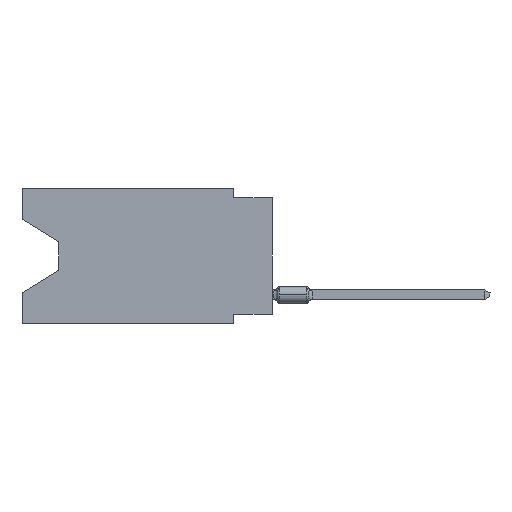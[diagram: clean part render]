
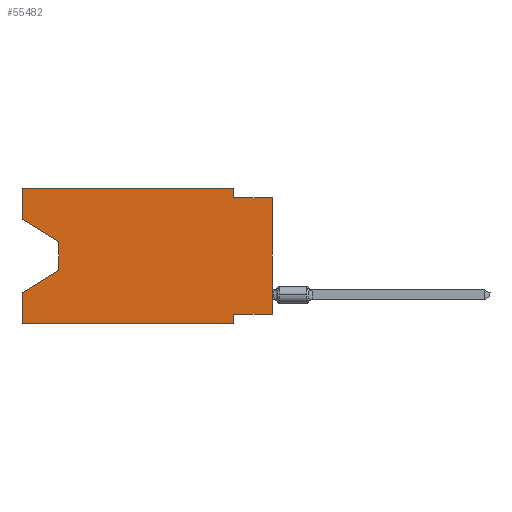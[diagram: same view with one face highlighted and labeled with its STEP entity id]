
A CAD part, left-side view. The second image highlights one B-rep face of the part: STEP entity #55482.
In plain terms, the highlighted planar face has unit normal (-1, 0, 0).
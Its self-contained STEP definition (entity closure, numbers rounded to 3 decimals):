
#681 = DIRECTION ( 'NONE',  ( 0., 0., -1. ) ) ;
#795 = CARTESIAN_POINT ( 'NONE',  ( 0., 16.383, 0. ) ) ;
#1353 = CARTESIAN_POINT ( 'NONE',  ( 0., 0., -0.635 ) ) ;
#1984 = EDGE_CURVE ( 'NONE', #32565, #71224, #25926, .T. ) ;
#2244 = CARTESIAN_POINT ( 'NONE',  ( 0., 16.383, 0. ) ) ;
#2328 = EDGE_LOOP ( 'NONE', ( #21225, #4674, #35212, #48874, #58972, #5348, #60784, #5587, #52796, #24719, #15482, #45468 ) ) ;
#2880 = CARTESIAN_POINT ( 'NONE',  ( 0., 2.54, -0.635 ) ) ;
#2923 = VERTEX_POINT ( 'NONE', #56044 ) ;
#3989 = CARTESIAN_POINT ( 'NONE',  ( 0., 16.383, -6.852 ) ) ;
#4352 = CARTESIAN_POINT ( 'NONE',  ( 0., 0., -8.255 ) ) ;
#4555 = CARTESIAN_POINT ( 'NONE',  ( 0., 16.383, -2.038 ) ) ;
#4674 = ORIENTED_EDGE ( 'NONE', *, *, #30506, .T. ) ;
#4693 = LINE ( 'NONE', #9456, #6741 ) ;
#5130 = VERTEX_POINT ( 'NONE', #795 ) ;
#5348 = ORIENTED_EDGE ( 'NONE', *, *, #31279, .F. ) ;
#5587 = ORIENTED_EDGE ( 'NONE', *, *, #11384, .T. ) ;
#5740 = VERTEX_POINT ( 'NONE', #2880 ) ;
#6534 = VECTOR ( 'NONE', #47181, 1000. ) ;
#6741 = VECTOR ( 'NONE', #36923, 1000. ) ;
#7385 = DIRECTION ( 'NONE',  ( 0., -1., 0. ) ) ;
#7559 = LINE ( 'NONE', #56991, #9021 ) ;
#7569 = LINE ( 'NONE', #13766, #56932 ) ;
#8771 = EDGE_CURVE ( 'NONE', #2923, #70282, #7569, .T. ) ;
#9021 = VECTOR ( 'NONE', #58058, 1000. ) ;
#9230 = EDGE_CURVE ( 'NONE', #18160, #30103, #10346, .T. ) ;
#9456 = CARTESIAN_POINT ( 'NONE',  ( 0., 0., 0. ) ) ;
#9576 = EDGE_CURVE ( 'NONE', #5130, #12371, #41776, .T. ) ;
#9900 = EDGE_CURVE ( 'NONE', #5740, #17515, #34660, .T. ) ;
#10346 = LINE ( 'NONE', #20239, #44099 ) ;
#11384 = EDGE_CURVE ( 'NONE', #32565, #17515, #4693, .T. ) ;
#12371 = VERTEX_POINT ( 'NONE', #15907 ) ;
#13766 = CARTESIAN_POINT ( 'NONE',  ( 0., 13.97, -5.385 ) ) ;
#15133 = CARTESIAN_POINT ( 'NONE',  ( 0., 16.383, -2.038 ) ) ;
#15482 = ORIENTED_EDGE ( 'NONE', *, *, #9576, .F. ) ;
#15907 = CARTESIAN_POINT ( 'NONE',  ( 0., 2.54, 0. ) ) ;
#16053 = DIRECTION ( 'NONE',  ( 0., 1., 0. ) ) ;
#16927 = EDGE_CURVE ( 'NONE', #40442, #5130, #27997, .T. ) ;
#17165 = DIRECTION ( 'NONE',  ( 1., 0., 0. ) ) ;
#17515 = VERTEX_POINT ( 'NONE', #32501 ) ;
#18089 = CARTESIAN_POINT ( 'NONE',  ( 0., 13.97, -3.505 ) ) ;
#18160 = VERTEX_POINT ( 'NONE', #64579 ) ;
#18292 = VECTOR ( 'NONE', #23671, 1000. ) ;
#20239 = CARTESIAN_POINT ( 'NONE',  ( 0., 16.383, -8.89 ) ) ;
#21225 = ORIENTED_EDGE ( 'NONE', *, *, #21826, .T. ) ;
#21410 = AXIS2_PLACEMENT_3D ( 'NONE', #29212, #17165, #681 ) ;
#21826 = EDGE_CURVE ( 'NONE', #40442, #34788, #53939, .T. ) ;
#23671 = DIRECTION ( 'NONE',  ( 0., -1., 0. ) ) ;
#24204 = VECTOR ( 'NONE', #67535, 1000. ) ;
#24719 = ORIENTED_EDGE ( 'NONE', *, *, #28900, .F. ) ;
#25926 = LINE ( 'NONE', #4352, #46910 ) ;
#26233 = CARTESIAN_POINT ( 'NONE',  ( 0., 2.54, -8.255 ) ) ;
#27997 = LINE ( 'NONE', #50331, #52174 ) ;
#28360 = DIRECTION ( 'NONE',  ( 0., 0., 1. ) ) ;
#28520 = CARTESIAN_POINT ( 'NONE',  ( 0., 2.54, -8.89 ) ) ;
#28900 = EDGE_CURVE ( 'NONE', #12371, #5740, #7559, .T. ) ;
#29212 = CARTESIAN_POINT ( 'NONE',  ( 0., 16.383, 0. ) ) ;
#30103 = VERTEX_POINT ( 'NONE', #28520 ) ;
#30506 = EDGE_CURVE ( 'NONE', #34788, #2923, #40070, .T. ) ;
#30897 = DIRECTION ( 'NONE',  ( 0., -0.855, -0.519 ) ) ;
#31279 = EDGE_CURVE ( 'NONE', #71224, #30103, #46106, .T. ) ;
#32501 = CARTESIAN_POINT ( 'NONE',  ( 0., 0., -0.635 ) ) ;
#32565 = VERTEX_POINT ( 'NONE', #71639 ) ;
#34660 = LINE ( 'NONE', #1353, #18292 ) ;
#34788 = VERTEX_POINT ( 'NONE', #69963 ) ;
#35212 = ORIENTED_EDGE ( 'NONE', *, *, #8771, .T. ) ;
#36923 = DIRECTION ( 'NONE',  ( 0., 0., 1. ) ) ;
#40070 = LINE ( 'NONE', #18089, #24204 ) ;
#40442 = VERTEX_POINT ( 'NONE', #4555 ) ;
#40583 = FACE_OUTER_BOUND ( 'NONE', #2328, .T. ) ;
#40615 = CARTESIAN_POINT ( 'NONE',  ( 0., 2.54, -8.89 ) ) ;
#41776 = LINE ( 'NONE', #2244, #68673 ) ;
#42299 = DIRECTION ( 'NONE',  ( 0., 0.855, -0.519 ) ) ;
#44099 = VECTOR ( 'NONE', #48055, 1000. ) ;
#44418 = VECTOR ( 'NONE', #30897, 1000. ) ;
#45468 = ORIENTED_EDGE ( 'NONE', *, *, #16927, .F. ) ;
#46106 = LINE ( 'NONE', #40615, #72242 ) ;
#46166 = EDGE_CURVE ( 'NONE', #18160, #70282, #53364, .T. ) ;
#46910 = VECTOR ( 'NONE', #16053, 1000. ) ;
#47181 = DIRECTION ( 'NONE',  ( 0., 0., 1. ) ) ;
#48055 = DIRECTION ( 'NONE',  ( 0., -1., 0. ) ) ;
#48874 = ORIENTED_EDGE ( 'NONE', *, *, #46166, .F. ) ;
#50331 = CARTESIAN_POINT ( 'NONE',  ( 0., 16.383, 0. ) ) ;
#52174 = VECTOR ( 'NONE', #28360, 1000. ) ;
#52796 = ORIENTED_EDGE ( 'NONE', *, *, #9900, .F. ) ;
#53364 = LINE ( 'NONE', #59221, #6534 ) ;
#53939 = LINE ( 'NONE', #15133, #44418 ) ;
#55482 = ADVANCED_FACE ( 'NONE', ( #40583 ), #61833, .F. ) ;
#56044 = CARTESIAN_POINT ( 'NONE',  ( 0., 13.97, -5.385 ) ) ;
#56932 = VECTOR ( 'NONE', #42299, 1000. ) ;
#56991 = CARTESIAN_POINT ( 'NONE',  ( 0., 2.54, 0. ) ) ;
#58058 = DIRECTION ( 'NONE',  ( 0., 0., -1. ) ) ;
#58972 = ORIENTED_EDGE ( 'NONE', *, *, #9230, .T. ) ;
#59221 = CARTESIAN_POINT ( 'NONE',  ( 0., 16.383, 0. ) ) ;
#60784 = ORIENTED_EDGE ( 'NONE', *, *, #1984, .F. ) ;
#61833 = PLANE ( 'NONE',  #21410 ) ;
#62949 = DIRECTION ( 'NONE',  ( 0., 0., -1. ) ) ;
#64579 = CARTESIAN_POINT ( 'NONE',  ( 0., 16.383, -8.89 ) ) ;
#67535 = DIRECTION ( 'NONE',  ( 0., 0., -1. ) ) ;
#68673 = VECTOR ( 'NONE', #7385, 1000. ) ;
#69963 = CARTESIAN_POINT ( 'NONE',  ( 0., 13.97, -3.505 ) ) ;
#70282 = VERTEX_POINT ( 'NONE', #3989 ) ;
#71224 = VERTEX_POINT ( 'NONE', #26233 ) ;
#71639 = CARTESIAN_POINT ( 'NONE',  ( 0., 0., -8.255 ) ) ;
#72242 = VECTOR ( 'NONE', #62949, 1000. ) ;
